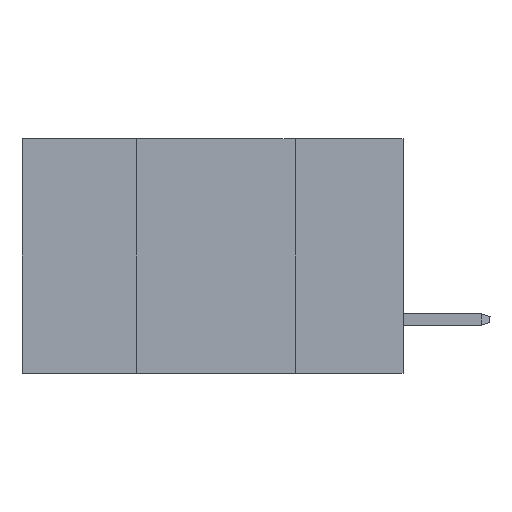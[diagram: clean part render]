
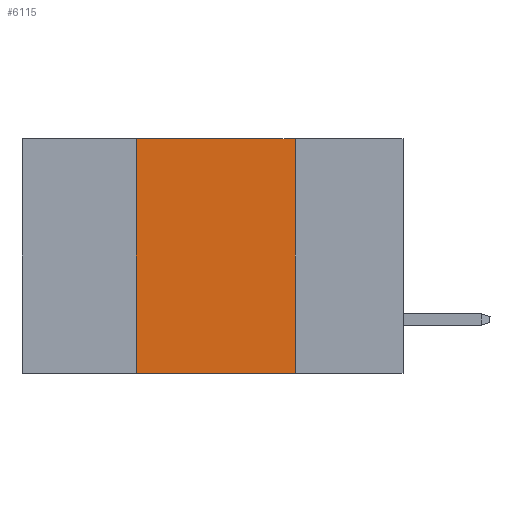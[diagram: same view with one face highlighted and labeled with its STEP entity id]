
A CAD part, left-side view. The second image highlights one B-rep face of the part: STEP entity #6115.
In plain terms, the highlighted planar face has unit normal (-1, 0, 0).
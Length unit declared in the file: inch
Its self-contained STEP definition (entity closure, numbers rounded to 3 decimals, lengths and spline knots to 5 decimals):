
#216 = VECTOR ( 'NONE', #20325, 39.37008 ) ;
#896 = VERTEX_POINT ( 'NONE', #9786 ) ;
#1041 = CARTESIAN_POINT ( 'NONE',  ( 0., 0.17, 0. ) ) ;
#1538 = EDGE_CURVE ( 'NONE', #17202, #17561, #5276, .T. ) ;
#1723 = FACE_OUTER_BOUND ( 'NONE', #4417, .T. ) ;
#1912 = CARTESIAN_POINT ( 'NONE',  ( 0., 0.42, 0. ) ) ;
#4417 = EDGE_LOOP ( 'NONE', ( #15620, #19562, #19132, #9911 ) ) ;
#5036 = LINE ( 'NONE', #11805, #216 ) ;
#5044 = VECTOR ( 'NONE', #10133, 39.37008 ) ;
#5276 = LINE ( 'NONE', #12046, #8208 ) ;
#6115 = ADVANCED_FACE ( 'NONE', ( #1723 ), #6844, .F. ) ;
#6252 = VECTOR ( 'NONE', #17906, 39.37008 ) ;
#6844 = PLANE ( 'NONE',  #10256 ) ;
#8208 = VECTOR ( 'NONE', #10157, 39.37008 ) ;
#8508 = DIRECTION ( 'NONE',  ( 1., 0., 0. ) ) ;
#9786 = CARTESIAN_POINT ( 'NONE',  ( 0., 0.17, -0.37 ) ) ;
#9911 = ORIENTED_EDGE ( 'NONE', *, *, #11213, .T. ) ;
#10133 = DIRECTION ( 'NONE',  ( 0., -1., 0. ) ) ;
#10157 = DIRECTION ( 'NONE',  ( 0., 0., 1. ) ) ;
#10256 = AXIS2_PLACEMENT_3D ( 'NONE', #13598, #8508, #20352 ) ;
#10833 = CARTESIAN_POINT ( 'NONE',  ( 0., 0.42, -0.37 ) ) ;
#11213 = EDGE_CURVE ( 'NONE', #17202, #896, #18779, .T. ) ;
#11805 = CARTESIAN_POINT ( 'NONE',  ( 0., 0.6, 0. ) ) ;
#12046 = CARTESIAN_POINT ( 'NONE',  ( 0., 0.42, 0. ) ) ;
#13563 = CARTESIAN_POINT ( 'NONE',  ( 0., 0.6, -0.37 ) ) ;
#13598 = CARTESIAN_POINT ( 'NONE',  ( 0., 0.6, 0. ) ) ;
#14694 = LINE ( 'NONE', #1041, #6252 ) ;
#15620 = ORIENTED_EDGE ( 'NONE', *, *, #16543, .F. ) ;
#16543 = EDGE_CURVE ( 'NONE', #16781, #896, #14694, .T. ) ;
#16781 = VERTEX_POINT ( 'NONE', #17289 ) ;
#17202 = VERTEX_POINT ( 'NONE', #10833 ) ;
#17289 = CARTESIAN_POINT ( 'NONE',  ( 0., 0.17, 0. ) ) ;
#17561 = VERTEX_POINT ( 'NONE', #1912 ) ;
#17906 = DIRECTION ( 'NONE',  ( 0., 0., -1. ) ) ;
#18779 = LINE ( 'NONE', #13563, #5044 ) ;
#19132 = ORIENTED_EDGE ( 'NONE', *, *, #1538, .F. ) ;
#19562 = ORIENTED_EDGE ( 'NONE', *, *, #20550, .F. ) ;
#20325 = DIRECTION ( 'NONE',  ( 0., -1., 0. ) ) ;
#20352 = DIRECTION ( 'NONE',  ( 0., 0., -1. ) ) ;
#20550 = EDGE_CURVE ( 'NONE', #17561, #16781, #5036, .T. ) ;
